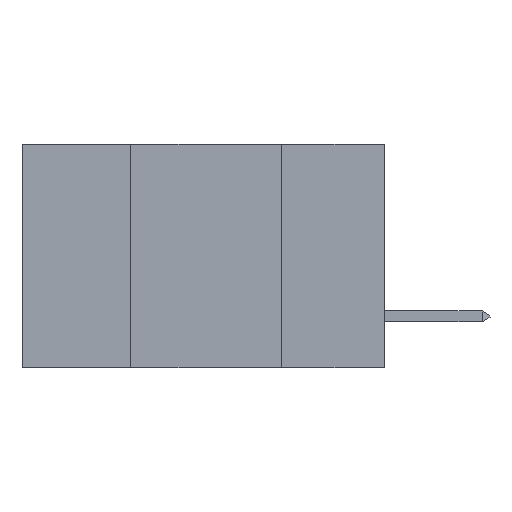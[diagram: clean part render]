
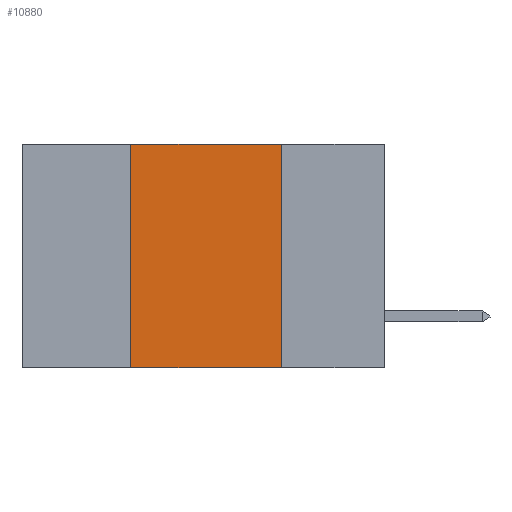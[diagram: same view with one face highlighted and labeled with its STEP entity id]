
A CAD part, left-side view. The second image highlights one B-rep face of the part: STEP entity #10880.
In plain terms, the highlighted planar face has unit normal (-1, 0, 0).
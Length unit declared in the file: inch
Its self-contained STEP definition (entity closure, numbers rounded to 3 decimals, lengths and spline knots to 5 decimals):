
#435 = CARTESIAN_POINT ( 'NONE',  ( 0., 0.6, 0. ) ) ;
#956 = DIRECTION ( 'NONE',  ( 0., 0., 1. ) ) ;
#1193 = VECTOR ( 'NONE', #14606, 39.37008 ) ;
#1585 = EDGE_CURVE ( 'NONE', #6665, #10427, #16800, .T. ) ;
#2048 = CARTESIAN_POINT ( 'NONE',  ( 0., 0.42, 0. ) ) ;
#2828 = DIRECTION ( 'NONE',  ( 1., 0., 0. ) ) ;
#3064 = DIRECTION ( 'NONE',  ( 0., -1., 0. ) ) ;
#3750 = VECTOR ( 'NONE', #956, 39.37008 ) ;
#5449 = LINE ( 'NONE', #19576, #1193 ) ;
#5661 = DIRECTION ( 'NONE',  ( 0., 0., -1. ) ) ;
#5954 = CARTESIAN_POINT ( 'NONE',  ( 0., 0.17, 0. ) ) ;
#6051 = AXIS2_PLACEMENT_3D ( 'NONE', #435, #2828, #7673 ) ;
#6643 = EDGE_CURVE ( 'NONE', #10427, #8499, #15732, .T. ) ;
#6665 = VERTEX_POINT ( 'NONE', #14595 ) ;
#7543 = ORIENTED_EDGE ( 'NONE', *, *, #12109, .F. ) ;
#7647 = ORIENTED_EDGE ( 'NONE', *, *, #1585, .F. ) ;
#7673 = DIRECTION ( 'NONE',  ( 0., 0., -1. ) ) ;
#8499 = VERTEX_POINT ( 'NONE', #13835 ) ;
#8787 = FACE_OUTER_BOUND ( 'NONE', #20494, .T. ) ;
#10427 = VERTEX_POINT ( 'NONE', #2048 ) ;
#10880 = ADVANCED_FACE ( 'NONE', ( #8787 ), #15032, .F. ) ;
#11057 = CARTESIAN_POINT ( 'NONE',  ( 0., 0.6, 0. ) ) ;
#11246 = LINE ( 'NONE', #5954, #12007 ) ;
#12007 = VECTOR ( 'NONE', #5661, 39.37008 ) ;
#12109 = EDGE_CURVE ( 'NONE', #8499, #17969, #11246, .T. ) ;
#13091 = CARTESIAN_POINT ( 'NONE',  ( 0., 0.17, -0.37 ) ) ;
#13835 = CARTESIAN_POINT ( 'NONE',  ( 0., 0.17, 0. ) ) ;
#14595 = CARTESIAN_POINT ( 'NONE',  ( 0., 0.42, -0.37 ) ) ;
#14606 = DIRECTION ( 'NONE',  ( 0., -1., 0. ) ) ;
#15032 = PLANE ( 'NONE',  #6051 ) ;
#15276 = CARTESIAN_POINT ( 'NONE',  ( 0., 0.42, 0. ) ) ;
#15732 = LINE ( 'NONE', #11057, #19948 ) ;
#16470 = ORIENTED_EDGE ( 'NONE', *, *, #17916, .T. ) ;
#16800 = LINE ( 'NONE', #15276, #3750 ) ;
#17916 = EDGE_CURVE ( 'NONE', #6665, #17969, #5449, .T. ) ;
#17969 = VERTEX_POINT ( 'NONE', #13091 ) ;
#19463 = ORIENTED_EDGE ( 'NONE', *, *, #6643, .F. ) ;
#19576 = CARTESIAN_POINT ( 'NONE',  ( 0., 0.6, -0.37 ) ) ;
#19948 = VECTOR ( 'NONE', #3064, 39.37008 ) ;
#20494 = EDGE_LOOP ( 'NONE', ( #7543, #19463, #7647, #16470 ) ) ;
